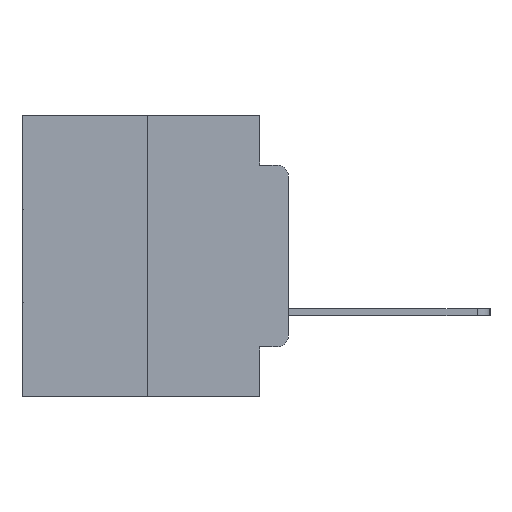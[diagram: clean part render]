
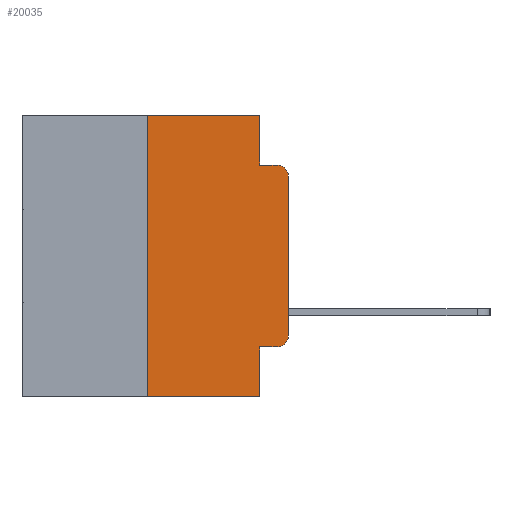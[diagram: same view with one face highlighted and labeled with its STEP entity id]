
A CAD part, left-side view. The second image highlights one B-rep face of the part: STEP entity #20035.
In plain terms, the highlighted planar face has unit normal (-1, 0, 0).
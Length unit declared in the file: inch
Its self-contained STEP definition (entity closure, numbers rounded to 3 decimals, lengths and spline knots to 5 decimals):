
#151 = LINE ( 'NONE', #16734, #5155 ) ;
#197 = ORIENTED_EDGE ( 'NONE', *, *, #21901, .T. ) ;
#234 = CARTESIAN_POINT ( 'NONE',  ( 0., 0.25, -0.5 ) ) ;
#516 = DIRECTION ( 'NONE',  ( 0., 0., -1. ) ) ;
#1076 = VERTEX_POINT ( 'NONE', #18641 ) ;
#1495 = EDGE_CURVE ( 'NONE', #14474, #20447, #11858, .T. ) ;
#1722 = VECTOR ( 'NONE', #10349, 39.37008 ) ;
#1803 = DIRECTION ( 'NONE',  ( 0., 0., -1. ) ) ;
#2662 = CARTESIAN_POINT ( 'NONE',  ( 0., 0.051, 0. ) ) ;
#3111 = VERTEX_POINT ( 'NONE', #3488 ) ;
#3191 = ORIENTED_EDGE ( 'NONE', *, *, #25988, .T. ) ;
#3488 = CARTESIAN_POINT ( 'NONE',  ( 0., 0.051, -0.4115 ) ) ;
#3736 = VERTEX_POINT ( 'NONE', #23051 ) ;
#4179 = ORIENTED_EDGE ( 'NONE', *, *, #9440, .T. ) ;
#4277 = DIRECTION ( 'NONE',  ( 0., -1., 0. ) ) ;
#4622 = DIRECTION ( 'NONE',  ( 0., 0., -1. ) ) ;
#4847 = DIRECTION ( 'NONE',  ( 1., 0., 0. ) ) ;
#4873 = CIRCLE ( 'NONE', #19275, 0.02 ) ;
#5100 = DIRECTION ( 'NONE',  ( 0., -1., 0. ) ) ;
#5155 = VECTOR ( 'NONE', #8224, 39.37008 ) ;
#5386 = EDGE_LOOP ( 'NONE', ( #4179, #11130, #22237, #7502, #13143, #19411, #3191, #25306, #15181, #197 ) ) ;
#5577 = VECTOR ( 'NONE', #4622, 39.37008 ) ;
#5848 = VECTOR ( 'NONE', #5100, 39.37008 ) ;
#6208 = VERTEX_POINT ( 'NONE', #9167 ) ;
#6824 = EDGE_CURVE ( 'NONE', #3111, #9110, #11474, .T. ) ;
#6888 = CARTESIAN_POINT ( 'NONE',  ( 0., 0.473, 0. ) ) ;
#7018 = DIRECTION ( 'NONE',  ( -1., 0., 0. ) ) ;
#7502 = ORIENTED_EDGE ( 'NONE', *, *, #1495, .F. ) ;
#7833 = VECTOR ( 'NONE', #4277, 39.37008 ) ;
#8139 = VECTOR ( 'NONE', #516, 39.37008 ) ;
#8224 = DIRECTION ( 'NONE',  ( 0., 0., 1. ) ) ;
#9110 = VERTEX_POINT ( 'NONE', #11329 ) ;
#9167 = CARTESIAN_POINT ( 'NONE',  ( 0., 0., -0.1085 ) ) ;
#9440 = EDGE_CURVE ( 'NONE', #22797, #6208, #24555, .T. ) ;
#10349 = DIRECTION ( 'NONE',  ( 0., 0., 1. ) ) ;
#10730 = FACE_OUTER_BOUND ( 'NONE', #5386, .T. ) ;
#11050 = EDGE_CURVE ( 'NONE', #3111, #3736, #13814, .T. ) ;
#11130 = ORIENTED_EDGE ( 'NONE', *, *, #18532, .T. ) ;
#11329 = CARTESIAN_POINT ( 'NONE',  ( 0., 0.02, -0.4115 ) ) ;
#11428 = EDGE_CURVE ( 'NONE', #20447, #18540, #24405, .T. ) ;
#11474 = LINE ( 'NONE', #13544, #5848 ) ;
#11858 = LINE ( 'NONE', #19912, #5577 ) ;
#13098 = EDGE_CURVE ( 'NONE', #1076, #14474, #18043, .T. ) ;
#13143 = ORIENTED_EDGE ( 'NONE', *, *, #13098, .F. ) ;
#13263 = DIRECTION ( 'NONE',  ( 0., -1., 0. ) ) ;
#13544 = CARTESIAN_POINT ( 'NONE',  ( 0., 0.051, -0.4115 ) ) ;
#13814 = LINE ( 'NONE', #2662, #8139 ) ;
#14474 = VERTEX_POINT ( 'NONE', #15428 ) ;
#14514 = DIRECTION ( 'NONE',  ( -1., 0., 0. ) ) ;
#15181 = ORIENTED_EDGE ( 'NONE', *, *, #6824, .T. ) ;
#15428 = CARTESIAN_POINT ( 'NONE',  ( 0., 0.051, 0. ) ) ;
#16729 = VECTOR ( 'NONE', #13263, 39.37008 ) ;
#16734 = CARTESIAN_POINT ( 'NONE',  ( 0., 0.25, 0. ) ) ;
#16969 = CIRCLE ( 'NONE', #23753, 0.02 ) ;
#17384 = DIRECTION ( 'NONE',  ( 0., -1., 0. ) ) ;
#17503 = CARTESIAN_POINT ( 'NONE',  ( 0., 0.473, 0. ) ) ;
#17591 = PLANE ( 'NONE',  #18107 ) ;
#17619 = CARTESIAN_POINT ( 'NONE',  ( 0., 0.02, -0.0885 ) ) ;
#18043 = LINE ( 'NONE', #6888, #16729 ) ;
#18107 = AXIS2_PLACEMENT_3D ( 'NONE', #17503, #4847, #19639 ) ;
#18393 = VECTOR ( 'NONE', #17384, 39.37008 ) ;
#18532 = EDGE_CURVE ( 'NONE', #6208, #18540, #4873, .T. ) ;
#18540 = VERTEX_POINT ( 'NONE', #17619 ) ;
#18631 = CARTESIAN_POINT ( 'NONE',  ( 0., 0.051, -0.0885 ) ) ;
#18641 = CARTESIAN_POINT ( 'NONE',  ( 0., 0.25, 0. ) ) ;
#19275 = AXIS2_PLACEMENT_3D ( 'NONE', #19667, #7018, #21677 ) ;
#19376 = CARTESIAN_POINT ( 'NONE',  ( 0., 0., -0.3915 ) ) ;
#19411 = ORIENTED_EDGE ( 'NONE', *, *, #19554, .F. ) ;
#19554 = EDGE_CURVE ( 'NONE', #24330, #1076, #151, .T. ) ;
#19639 = DIRECTION ( 'NONE',  ( 0., 0., -1. ) ) ;
#19667 = CARTESIAN_POINT ( 'NONE',  ( 0., 0.02, -0.1085 ) ) ;
#19912 = CARTESIAN_POINT ( 'NONE',  ( 0., 0.051, 0. ) ) ;
#20035 = ADVANCED_FACE ( 'NONE', ( #10730 ), #17591, .F. ) ;
#20447 = VERTEX_POINT ( 'NONE', #18631 ) ;
#20952 = CARTESIAN_POINT ( 'NONE',  ( 0., 0., 0. ) ) ;
#21677 = DIRECTION ( 'NONE',  ( 0., 0., -1. ) ) ;
#21901 = EDGE_CURVE ( 'NONE', #9110, #22797, #16969, .T. ) ;
#22237 = ORIENTED_EDGE ( 'NONE', *, *, #11428, .F. ) ;
#22797 = VERTEX_POINT ( 'NONE', #19376 ) ;
#23051 = CARTESIAN_POINT ( 'NONE',  ( 0., 0.051, -0.5 ) ) ;
#23718 = LINE ( 'NONE', #25336, #18393 ) ;
#23753 = AXIS2_PLACEMENT_3D ( 'NONE', #26640, #14514, #1803 ) ;
#24330 = VERTEX_POINT ( 'NONE', #234 ) ;
#24405 = LINE ( 'NONE', #25006, #7833 ) ;
#24555 = LINE ( 'NONE', #20952, #1722 ) ;
#25006 = CARTESIAN_POINT ( 'NONE',  ( 0., 0.051, -0.0885 ) ) ;
#25306 = ORIENTED_EDGE ( 'NONE', *, *, #11050, .F. ) ;
#25336 = CARTESIAN_POINT ( 'NONE',  ( 0., 0.473, -0.5 ) ) ;
#25988 = EDGE_CURVE ( 'NONE', #24330, #3736, #23718, .T. ) ;
#26640 = CARTESIAN_POINT ( 'NONE',  ( 0., 0.02, -0.3915 ) ) ;
